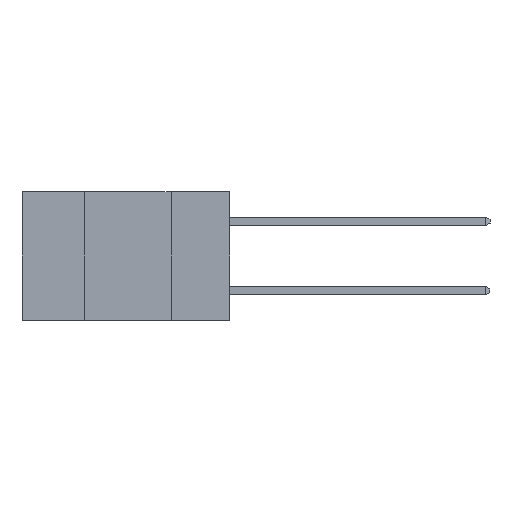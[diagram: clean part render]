
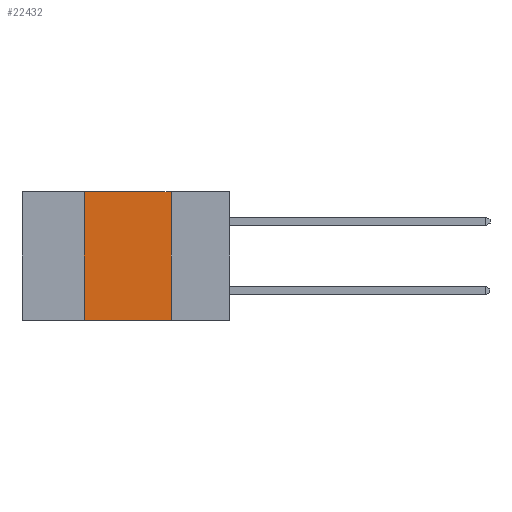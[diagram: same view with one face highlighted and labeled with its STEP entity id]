
A CAD part, left-side view. The second image highlights one B-rep face of the part: STEP entity #22432.
In plain terms, the highlighted planar face has unit normal (-1, 0, 0).
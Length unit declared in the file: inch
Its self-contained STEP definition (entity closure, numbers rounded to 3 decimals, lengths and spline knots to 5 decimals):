
#1055 = EDGE_LOOP ( 'NONE', ( #6301, #2638, #12361, #17160 ) ) ;
#1061 = CARTESIAN_POINT ( 'NONE',  ( 0., 0.6, 0. ) ) ;
#1436 = CARTESIAN_POINT ( 'NONE',  ( 0., 0.6, 0. ) ) ;
#1620 = LINE ( 'NONE', #1061, #6448 ) ;
#2638 = ORIENTED_EDGE ( 'NONE', *, *, #17132, .F. ) ;
#2820 = CARTESIAN_POINT ( 'NONE',  ( 0., 0.42, -0.37 ) ) ;
#3294 = DIRECTION ( 'NONE',  ( 0., 0., -1. ) ) ;
#3617 = DIRECTION ( 'NONE',  ( 0., 0., 1. ) ) ;
#3708 = CARTESIAN_POINT ( 'NONE',  ( 0., 0.42, 0. ) ) ;
#4707 = DIRECTION ( 'NONE',  ( 0., -1., 0. ) ) ;
#6301 = ORIENTED_EDGE ( 'NONE', *, *, #9108, .F. ) ;
#6448 = VECTOR ( 'NONE', #4707, 39.37008 ) ;
#6824 = PLANE ( 'NONE',  #7496 ) ;
#7259 = EDGE_CURVE ( 'NONE', #10301, #22599, #19381, .T. ) ;
#7312 = LINE ( 'NONE', #23326, #20682 ) ;
#7380 = VECTOR ( 'NONE', #3617, 39.37008 ) ;
#7406 = VECTOR ( 'NONE', #9300, 39.37008 ) ;
#7496 = AXIS2_PLACEMENT_3D ( 'NONE', #1436, #14250, #3294 ) ;
#7720 = EDGE_CURVE ( 'NONE', #10301, #14515, #12283, .T. ) ;
#8505 = CARTESIAN_POINT ( 'NONE',  ( 0., 0.17, 0. ) ) ;
#9108 = EDGE_CURVE ( 'NONE', #17990, #22599, #7312, .T. ) ;
#9300 = DIRECTION ( 'NONE',  ( 0., -1., 0. ) ) ;
#9350 = CARTESIAN_POINT ( 'NONE',  ( 0., 0.6, -0.37 ) ) ;
#10301 = VERTEX_POINT ( 'NONE', #2820 ) ;
#12283 = LINE ( 'NONE', #3708, #7380 ) ;
#12361 = ORIENTED_EDGE ( 'NONE', *, *, #7720, .F. ) ;
#14162 = FACE_OUTER_BOUND ( 'NONE', #1055, .T. ) ;
#14250 = DIRECTION ( 'NONE',  ( 1., 0., 0. ) ) ;
#14515 = VERTEX_POINT ( 'NONE', #22624 ) ;
#16174 = DIRECTION ( 'NONE',  ( 0., 0., -1. ) ) ;
#17132 = EDGE_CURVE ( 'NONE', #14515, #17990, #1620, .T. ) ;
#17160 = ORIENTED_EDGE ( 'NONE', *, *, #7259, .T. ) ;
#17990 = VERTEX_POINT ( 'NONE', #8505 ) ;
#18243 = CARTESIAN_POINT ( 'NONE',  ( 0., 0.17, -0.37 ) ) ;
#19381 = LINE ( 'NONE', #9350, #7406 ) ;
#20682 = VECTOR ( 'NONE', #16174, 39.37008 ) ;
#22432 = ADVANCED_FACE ( 'NONE', ( #14162 ), #6824, .F. ) ;
#22599 = VERTEX_POINT ( 'NONE', #18243 ) ;
#22624 = CARTESIAN_POINT ( 'NONE',  ( 0., 0.42, 0. ) ) ;
#23326 = CARTESIAN_POINT ( 'NONE',  ( 0., 0.17, 0. ) ) ;
